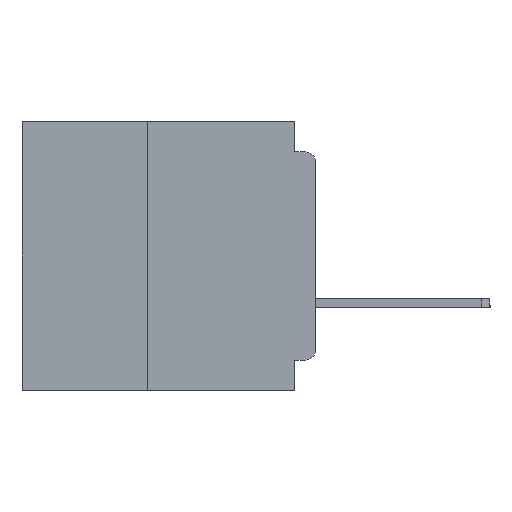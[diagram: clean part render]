
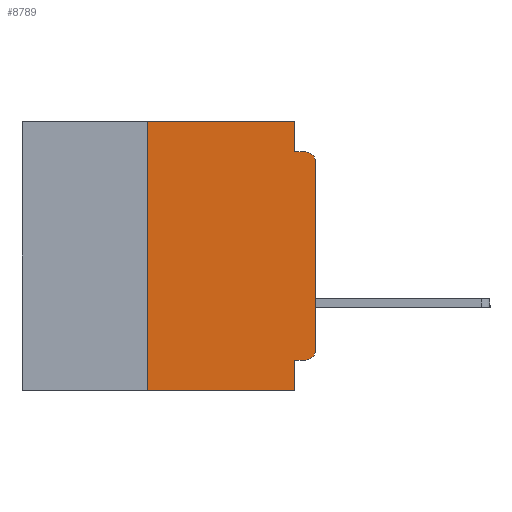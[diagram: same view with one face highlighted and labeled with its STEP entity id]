
A CAD part, left-side view. The second image highlights one B-rep face of the part: STEP entity #8789.
In plain terms, the highlighted planar face has unit normal (-1, 0, 0).
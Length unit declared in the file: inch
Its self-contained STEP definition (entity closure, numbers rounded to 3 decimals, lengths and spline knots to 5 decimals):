
#2710 = FACE_OUTER_BOUND ( 'NONE', #67400, .T. ) ;
#3176 = EDGE_CURVE ( 'NONE', #20479, #63906, #6811, .T. ) ;
#3535 = VERTEX_POINT ( 'NONE', #32736 ) ;
#4230 = CARTESIAN_POINT ( 'NONE',  ( 0., 0., -0.06 ) ) ;
#4460 = ORIENTED_EDGE ( 'NONE', *, *, #37650, .F. ) ;
#4984 = CARTESIAN_POINT ( 'NONE',  ( 0., 0.437, 0. ) ) ;
#6811 = CIRCLE ( 'NONE', #47915, 0.015 ) ;
#6815 = LINE ( 'NONE', #4984, #33671 ) ;
#8387 = PLANE ( 'NONE',  #62982 ) ;
#8789 = ADVANCED_FACE ( 'NONE', ( #2710 ), #8387, .F. ) ;
#10388 = DIRECTION ( 'NONE',  ( 0., -1., 0. ) ) ;
#11194 = LINE ( 'NONE', #55460, #38116 ) ;
#12567 = ORIENTED_EDGE ( 'NONE', *, *, #15650, .F. ) ;
#13138 = ORIENTED_EDGE ( 'NONE', *, *, #3176, .T. ) ;
#15650 = EDGE_CURVE ( 'NONE', #3535, #56034, #41353, .T. ) ;
#17121 = VECTOR ( 'NONE', #66899, 39.37008 ) ;
#19185 = DIRECTION ( 'NONE',  ( 0., 0., -1. ) ) ;
#19197 = ORIENTED_EDGE ( 'NONE', *, *, #57979, .F. ) ;
#20479 = VERTEX_POINT ( 'NONE', #46715 ) ;
#21760 = CARTESIAN_POINT ( 'NONE',  ( 0., 0.015, -0.045 ) ) ;
#22290 = ORIENTED_EDGE ( 'NONE', *, *, #56854, .T. ) ;
#22460 = VERTEX_POINT ( 'NONE', #33335 ) ;
#23669 = VECTOR ( 'NONE', #36483, 39.37008 ) ;
#25159 = CARTESIAN_POINT ( 'NONE',  ( 0., 0., -0.355 ) ) ;
#25889 = VERTEX_POINT ( 'NONE', #4230 ) ;
#26329 = VECTOR ( 'NONE', #67595, 39.37008 ) ;
#26704 = CARTESIAN_POINT ( 'NONE',  ( 0., 0.015, -0.34 ) ) ;
#26751 = CARTESIAN_POINT ( 'NONE',  ( 0., 0.031, -0.355 ) ) ;
#27084 = VECTOR ( 'NONE', #62272, 39.37008 ) ;
#29412 = CIRCLE ( 'NONE', #47194, 0.015 ) ;
#29508 = CARTESIAN_POINT ( 'NONE',  ( 0., 0.015, -0.06 ) ) ;
#31040 = CARTESIAN_POINT ( 'NONE',  ( 0., 0.437, -0.4 ) ) ;
#32060 = DIRECTION ( 'NONE',  ( 0., 0., -1. ) ) ;
#32736 = CARTESIAN_POINT ( 'NONE',  ( 0., 0.031, 0. ) ) ;
#33333 = ORIENTED_EDGE ( 'NONE', *, *, #67411, .F. ) ;
#33335 = CARTESIAN_POINT ( 'NONE',  ( 0., 0.25, -0.4 ) ) ;
#33671 = VECTOR ( 'NONE', #10388, 39.37008 ) ;
#34130 = EDGE_CURVE ( 'NONE', #63906, #25889, #59810, .T. ) ;
#34894 = CARTESIAN_POINT ( 'NONE',  ( 0., 0., 0. ) ) ;
#34921 = DIRECTION ( 'NONE',  ( 0., 0., -1. ) ) ;
#35300 = ORIENTED_EDGE ( 'NONE', *, *, #67617, .F. ) ;
#35388 = EDGE_CURVE ( 'NONE', #22460, #46562, #52163, .T. ) ;
#35768 = CARTESIAN_POINT ( 'NONE',  ( 0., 0., -0.34 ) ) ;
#35992 = VECTOR ( 'NONE', #48153, 39.37008 ) ;
#36126 = VERTEX_POINT ( 'NONE', #52972 ) ;
#36178 = DIRECTION ( 'NONE',  ( 0., 1., 0. ) ) ;
#36483 = DIRECTION ( 'NONE',  ( 0., -1., 0. ) ) ;
#36768 = ORIENTED_EDGE ( 'NONE', *, *, #34130, .T. ) ;
#37650 = EDGE_CURVE ( 'NONE', #36126, #3535, #6815, .T. ) ;
#38116 = VECTOR ( 'NONE', #60804, 39.37008 ) ;
#39241 = VECTOR ( 'NONE', #36178, 39.37008 ) ;
#39920 = EDGE_CURVE ( 'NONE', #20479, #59097, #67630, .T. ) ;
#41353 = LINE ( 'NONE', #46155, #27084 ) ;
#43956 = VERTEX_POINT ( 'NONE', #21760 ) ;
#45859 = CARTESIAN_POINT ( 'NONE',  ( 0., 0.437, 0. ) ) ;
#46155 = CARTESIAN_POINT ( 'NONE',  ( 0., 0.031, 0. ) ) ;
#46562 = VERTEX_POINT ( 'NONE', #67251 ) ;
#46715 = CARTESIAN_POINT ( 'NONE',  ( 0., 0.015, -0.355 ) ) ;
#47194 = AXIS2_PLACEMENT_3D ( 'NONE', #29508, #66925, #34921 ) ;
#47915 = AXIS2_PLACEMENT_3D ( 'NONE', #26704, #64085, #32060 ) ;
#47919 = CARTESIAN_POINT ( 'NONE',  ( 0., 0.031, -0.4 ) ) ;
#48153 = DIRECTION ( 'NONE',  ( 0., 0., -1. ) ) ;
#50158 = LINE ( 'NONE', #47919, #35992 ) ;
#51269 = DIRECTION ( 'NONE',  ( 1., 0., 0. ) ) ;
#52163 = LINE ( 'NONE', #31040, #23669 ) ;
#52972 = CARTESIAN_POINT ( 'NONE',  ( 0., 0.25, 0. ) ) ;
#55460 = CARTESIAN_POINT ( 'NONE',  ( 0., 0.25, -0.4 ) ) ;
#56034 = VERTEX_POINT ( 'NONE', #63983 ) ;
#56854 = EDGE_CURVE ( 'NONE', #25889, #43956, #29412, .T. ) ;
#57979 = EDGE_CURVE ( 'NONE', #59097, #46562, #50158, .T. ) ;
#59097 = VERTEX_POINT ( 'NONE', #26751 ) ;
#59810 = LINE ( 'NONE', #34894, #17121 ) ;
#60804 = DIRECTION ( 'NONE',  ( 0., 0., 1. ) ) ;
#62207 = CARTESIAN_POINT ( 'NONE',  ( 0., 0., -0.045 ) ) ;
#62272 = DIRECTION ( 'NONE',  ( 0., 0., -1. ) ) ;
#62982 = AXIS2_PLACEMENT_3D ( 'NONE', #45859, #51269, #19185 ) ;
#63906 = VERTEX_POINT ( 'NONE', #35768 ) ;
#63915 = ORIENTED_EDGE ( 'NONE', *, *, #39920, .F. ) ;
#63983 = CARTESIAN_POINT ( 'NONE',  ( 0., 0.031, -0.045 ) ) ;
#64085 = DIRECTION ( 'NONE',  ( -1., 0., 0. ) ) ;
#66899 = DIRECTION ( 'NONE',  ( 0., 0., 1. ) ) ;
#66925 = DIRECTION ( 'NONE',  ( -1., 0., 0. ) ) ;
#67251 = CARTESIAN_POINT ( 'NONE',  ( 0., 0.031, -0.4 ) ) ;
#67400 = EDGE_LOOP ( 'NONE', ( #36768, #22290, #35300, #12567, #4460, #33333, #67654, #19197, #63915, #13138 ) ) ;
#67411 = EDGE_CURVE ( 'NONE', #22460, #36126, #11194, .T. ) ;
#67595 = DIRECTION ( 'NONE',  ( 0., -1., 0. ) ) ;
#67617 = EDGE_CURVE ( 'NONE', #56034, #43956, #68977, .T. ) ;
#67630 = LINE ( 'NONE', #25159, #39241 ) ;
#67654 = ORIENTED_EDGE ( 'NONE', *, *, #35388, .T. ) ;
#68977 = LINE ( 'NONE', #62207, #26329 ) ;
